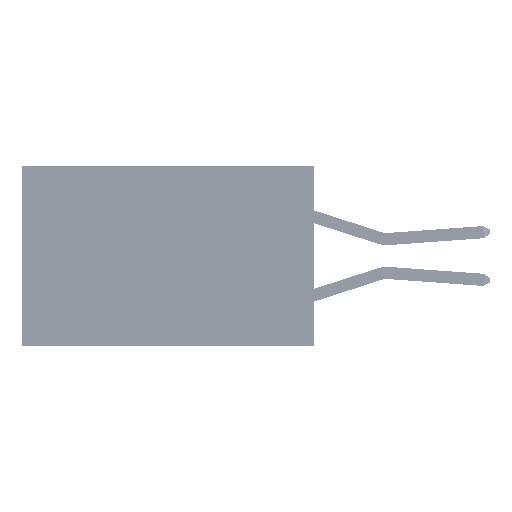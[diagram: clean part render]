
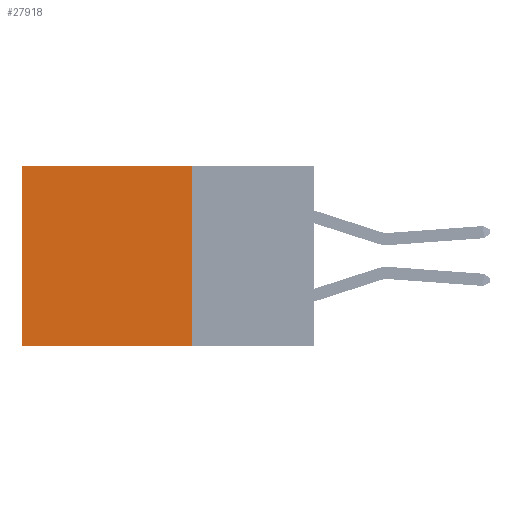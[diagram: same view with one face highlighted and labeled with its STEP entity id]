
A CAD part, left-side view. The second image highlights one B-rep face of the part: STEP entity #27918.
In plain terms, the highlighted planar face has unit normal (-1, 0, 0).
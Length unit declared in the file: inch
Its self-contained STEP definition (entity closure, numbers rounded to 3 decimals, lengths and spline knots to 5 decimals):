
#1009 = CARTESIAN_POINT ( 'NONE',  ( 0.2875, 0.25, 0. ) ) ;
#1614 = EDGE_CURVE ( 'NONE', #33034, #43111, #18736, .T. ) ;
#2301 = EDGE_CURVE ( 'NONE', #29239, #43111, #40349, .T. ) ;
#2337 = CARTESIAN_POINT ( 'NONE',  ( 0.2875, 0.25, -0.37 ) ) ;
#3337 = DIRECTION ( 'NONE',  ( 0., 0., -1. ) ) ;
#4482 = VECTOR ( 'NONE', #41163, 39.37008 ) ;
#4935 = LINE ( 'NONE', #8165, #4482 ) ;
#6627 = AXIS2_PLACEMENT_3D ( 'NONE', #1009, #38016, #42568 ) ;
#8165 = CARTESIAN_POINT ( 'NONE',  ( 0.2875, 0.25, 0. ) ) ;
#8424 = EDGE_CURVE ( 'NONE', #40649, #29239, #47420, .T. ) ;
#11054 = EDGE_CURVE ( 'NONE', #40649, #33034, #4935, .T. ) ;
#16508 = ORIENTED_EDGE ( 'NONE', *, *, #11054, .F. ) ;
#18736 = LINE ( 'NONE', #2337, #25607 ) ;
#19027 = VECTOR ( 'NONE', #30510, 39.37008 ) ;
#20321 = EDGE_LOOP ( 'NONE', ( #20392, #26632, #16508, #47997 ) ) ;
#20392 = ORIENTED_EDGE ( 'NONE', *, *, #2301, .T. ) ;
#24607 = VECTOR ( 'NONE', #3337, 39.37008 ) ;
#25607 = VECTOR ( 'NONE', #35050, 39.37008 ) ;
#26632 = ORIENTED_EDGE ( 'NONE', *, *, #1614, .F. ) ;
#27918 = ADVANCED_FACE ( 'NONE', ( #44780 ), #28684, .F. ) ;
#28684 = PLANE ( 'NONE',  #6627 ) ;
#29239 = VERTEX_POINT ( 'NONE', #35985 ) ;
#30510 = DIRECTION ( 'NONE',  ( 0., 1., 0. ) ) ;
#33034 = VERTEX_POINT ( 'NONE', #48555 ) ;
#33730 = CARTESIAN_POINT ( 'NONE',  ( 0.2875, 0.25, 0. ) ) ;
#35050 = DIRECTION ( 'NONE',  ( 0., 1., 0. ) ) ;
#35985 = CARTESIAN_POINT ( 'NONE',  ( 0.2875, 0.6, 0. ) ) ;
#38016 = DIRECTION ( 'NONE',  ( 1., 0., 0. ) ) ;
#39754 = CARTESIAN_POINT ( 'NONE',  ( 0.2875, 0.6, -0.37 ) ) ;
#40349 = LINE ( 'NONE', #44132, #24607 ) ;
#40649 = VERTEX_POINT ( 'NONE', #33730 ) ;
#41163 = DIRECTION ( 'NONE',  ( 0., 0., -1. ) ) ;
#42568 = DIRECTION ( 'NONE',  ( 0., 0., -1. ) ) ;
#43111 = VERTEX_POINT ( 'NONE', #39754 ) ;
#43652 = CARTESIAN_POINT ( 'NONE',  ( 0.2875, 0.25, 0. ) ) ;
#44132 = CARTESIAN_POINT ( 'NONE',  ( 0.2875, 0.6, 0. ) ) ;
#44780 = FACE_OUTER_BOUND ( 'NONE', #20321, .T. ) ;
#47420 = LINE ( 'NONE', #43652, #19027 ) ;
#47997 = ORIENTED_EDGE ( 'NONE', *, *, #8424, .T. ) ;
#48555 = CARTESIAN_POINT ( 'NONE',  ( 0.2875, 0.25, -0.37 ) ) ;
